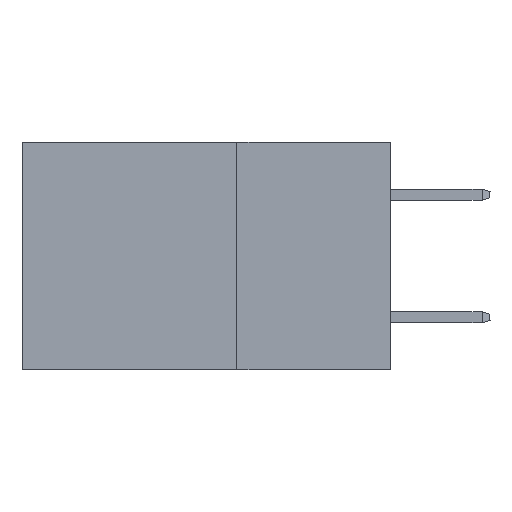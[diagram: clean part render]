
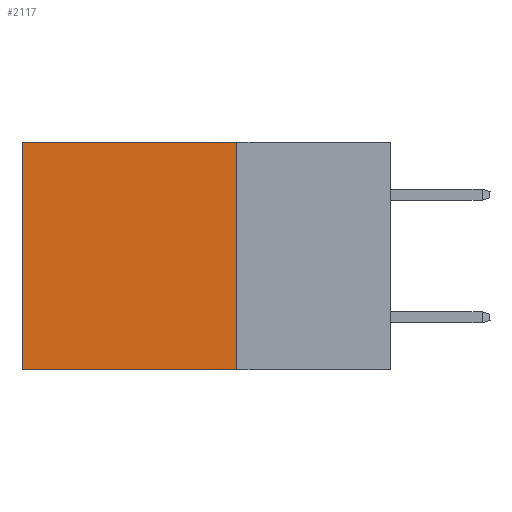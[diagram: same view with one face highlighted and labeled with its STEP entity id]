
A CAD part, left-side view. The second image highlights one B-rep face of the part: STEP entity #2117.
In plain terms, the highlighted planar face has unit normal (-1, 0, 0).
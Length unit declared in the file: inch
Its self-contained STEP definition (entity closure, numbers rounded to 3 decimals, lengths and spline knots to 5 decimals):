
#662 = LINE ( 'NONE', #34438, #43205 ) ;
#1010 = DIRECTION ( 'NONE',  ( 0., 1., 0. ) ) ;
#1745 = VERTEX_POINT ( 'NONE', #22631 ) ;
#2117 = ADVANCED_FACE ( 'NONE', ( #27374 ), #34682, .F. ) ;
#2165 = VECTOR ( 'NONE', #29491, 39.37008 ) ;
#3327 = VERTEX_POINT ( 'NONE', #8537 ) ;
#3711 = LINE ( 'NONE', #9159, #2165 ) ;
#6634 = CARTESIAN_POINT ( 'NONE',  ( 0.2875, 0.25, 0. ) ) ;
#8537 = CARTESIAN_POINT ( 'NONE',  ( 0.2875, 0.6, -0.37 ) ) ;
#8994 = DIRECTION ( 'NONE',  ( 0., 1., 0. ) ) ;
#9159 = CARTESIAN_POINT ( 'NONE',  ( 0.2875, 0.6, 0. ) ) ;
#11869 = CARTESIAN_POINT ( 'NONE',  ( 0.2875, 0.25, 0. ) ) ;
#12486 = ORIENTED_EDGE ( 'NONE', *, *, #16619, .T. ) ;
#12670 = CARTESIAN_POINT ( 'NONE',  ( 0.2875, 0.6, 0. ) ) ;
#12989 = ORIENTED_EDGE ( 'NONE', *, *, #22070, .F. ) ;
#13991 = VERTEX_POINT ( 'NONE', #12670 ) ;
#16317 = LINE ( 'NONE', #39759, #23130 ) ;
#16430 = AXIS2_PLACEMENT_3D ( 'NONE', #11869, #35219, #19509 ) ;
#16619 = EDGE_CURVE ( 'NONE', #36950, #13991, #662, .T. ) ;
#18218 = ORIENTED_EDGE ( 'NONE', *, *, #27373, .F. ) ;
#19509 = DIRECTION ( 'NONE',  ( 0., 0., -1. ) ) ;
#20154 = ORIENTED_EDGE ( 'NONE', *, *, #36830, .T. ) ;
#22070 = EDGE_CURVE ( 'NONE', #1745, #3327, #16317, .T. ) ;
#22631 = CARTESIAN_POINT ( 'NONE',  ( 0.2875, 0.25, -0.37 ) ) ;
#23130 = VECTOR ( 'NONE', #8994, 39.37008 ) ;
#24514 = CARTESIAN_POINT ( 'NONE',  ( 0.2875, 0.25, 0. ) ) ;
#26888 = EDGE_LOOP ( 'NONE', ( #20154, #12989, #18218, #12486 ) ) ;
#27373 = EDGE_CURVE ( 'NONE', #36950, #1745, #42639, .T. ) ;
#27374 = FACE_OUTER_BOUND ( 'NONE', #26888, .T. ) ;
#28988 = VECTOR ( 'NONE', #31221, 39.37008 ) ;
#29491 = DIRECTION ( 'NONE',  ( 0., 0., -1. ) ) ;
#31221 = DIRECTION ( 'NONE',  ( 0., 0., -1. ) ) ;
#34438 = CARTESIAN_POINT ( 'NONE',  ( 0.2875, 0.25, 0. ) ) ;
#34682 = PLANE ( 'NONE',  #16430 ) ;
#35219 = DIRECTION ( 'NONE',  ( 1., 0., 0. ) ) ;
#36830 = EDGE_CURVE ( 'NONE', #13991, #3327, #3711, .T. ) ;
#36950 = VERTEX_POINT ( 'NONE', #6634 ) ;
#39759 = CARTESIAN_POINT ( 'NONE',  ( 0.2875, 0.25, -0.37 ) ) ;
#42639 = LINE ( 'NONE', #24514, #28988 ) ;
#43205 = VECTOR ( 'NONE', #1010, 39.37008 ) ;
